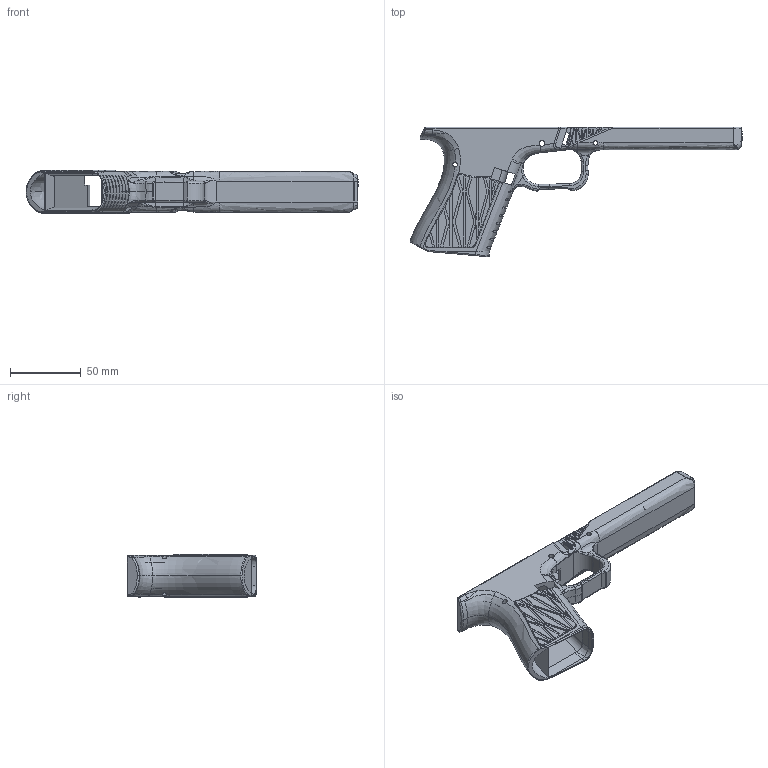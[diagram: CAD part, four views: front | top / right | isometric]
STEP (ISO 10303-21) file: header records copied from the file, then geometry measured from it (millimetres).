
FILE_DESCRIPTION(/* description */ (''),/* implementation_level */ '2;1');
FILE_NAME(/* name */ 'LB17 Frame Stippled V1.step',/* time_stamp */ '2021-02-22T13:27:40-07:00',/* author */ (''),/* organization */ (''),/* preprocessor_version */ 'ST-DEVELOPER v18.1',/* originating_system */ 'Autodesk Translation Framework v9.7.1.1290',/* authorisation */ '');
FILE_SCHEMA (('AUTOMOTIVE_DESIGN { 1 0 10303 214 3 1 1 }'));
Products named in the file (1): LB17 Frame Stippled
Bounding box: 235.25 x 91.73 x 30.6 mm (x, y, z)
Volume: 95996.8 mm3; surface area: 51932.3 mm2
Topology: 1 solids, 1 shells, 1305 faces, 3549 edges, 2224 vertices
Faces by surface type: bspline 603, plane 561, cylinder 121, torus 15, sphere 5
Full cylindrical faces by diameter (mm): 1.5 x2, 3.225 x2, 3.25 x2, 4.05 x2
Entity records: 79135 total; most frequent: CARTESIAN_POINT 51587, ORIENTED_EDGE 7078, DIRECTION 3961, EDGE_CURVE 3539, VERTEX_POINT 2224, LINE 1871, VECTOR 1871, EDGE_LOOP 1321
